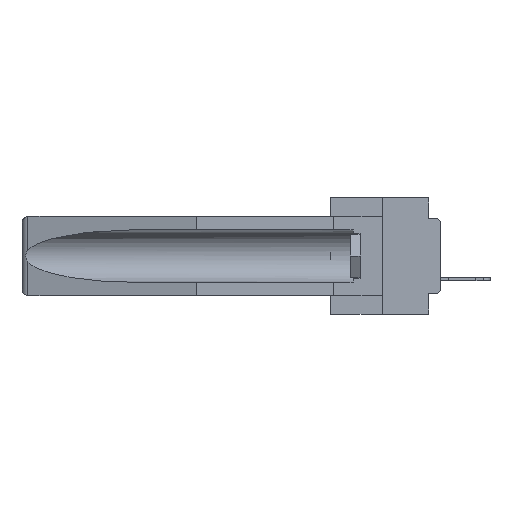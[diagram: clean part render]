
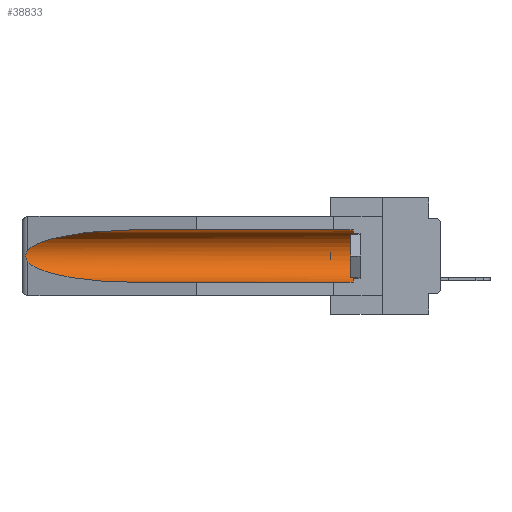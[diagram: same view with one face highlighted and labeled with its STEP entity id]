
A CAD part, left-side view. The second image highlights one B-rep face of the part: STEP entity #38833.
In plain terms, the highlighted cylindrical face has radius 2.857 mm (diameter 5.715 mm), a partial arc.
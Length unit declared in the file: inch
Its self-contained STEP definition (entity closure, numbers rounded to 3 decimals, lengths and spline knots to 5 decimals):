
#16 = LINE ( 'NONE', #34890, #8395 ) ;
#992 = CARTESIAN_POINT ( 'NONE',  ( 0.155, 0.126, -0.1715 ) ) ;
#1209 = EDGE_CURVE ( 'NONE', #10448, #9523, #7108, .T. ) ;
#2883 = VERTEX_POINT ( 'NONE', #7000 ) ;
#3504 = CARTESIAN_POINT ( 'NONE',  ( 0.25451, 1.48313, -0.09465 ) ) ;
#4136 = ORIENTED_EDGE ( 'NONE', *, *, #5567, .T. ) ;
#4322 = CARTESIAN_POINT ( 'NONE',  ( 0.26654, 1.53092, -0.15636 ) ) ;
#4549 = VECTOR ( 'NONE', #17404, 39.37008 ) ;
#5567 = EDGE_CURVE ( 'NONE', #2883, #10448, #33240, .T. ) ;
#6249 = DIRECTION ( 'NONE',  ( 0., 0., 1. ) ) ;
#6333 = VERTEX_POINT ( 'NONE', #38451 ) ;
#6442 = ORIENTED_EDGE ( 'NONE', *, *, #27187, .T. ) ;
#6509 = CARTESIAN_POINT ( 'NONE',  ( 0.155, -0.30754, -0.1715 ) ) ;
#7000 = CARTESIAN_POINT ( 'NONE',  ( 0.155, 1.07973, -0.059 ) ) ;
#7108 = B_SPLINE_CURVE_WITH_KNOTS ( 'NONE', 3,
 ( #26127, #9974, #4322, #22998, #35329, #26265, #19696, #31904, #32037, #7487 ),
 .UNSPECIFIED., .F., .F.,
 ( 4, 2, 2, 2, 4 ),
 ( 0., 0.00029, 0.00058, 0.00087, 0.00117 ),
 .UNSPECIFIED. ) ;
#7487 = CARTESIAN_POINT ( 'NONE',  ( 0.26537, 1.52718, -0.19328 ) ) ;
#7825 = CARTESIAN_POINT ( 'NONE',  ( 0.155, -0.30754, -0.059 ) ) ;
#8395 = VECTOR ( 'NONE', #31593, 39.37008 ) ;
#9523 = VERTEX_POINT ( 'NONE', #29130 ) ;
#9845 = CARTESIAN_POINT ( 'NONE',  ( 0.26537, 1.52718, -0.14972 ) ) ;
#9974 = CARTESIAN_POINT ( 'NONE',  ( 0.26597, 1.52961, -0.15275 ) ) ;
#10448 = VERTEX_POINT ( 'NONE', #27277 ) ;
#11919 = LINE ( 'NONE', #7825, #4549 ) ;
#12287 = EDGE_LOOP ( 'NONE', ( #4136, #14485, #6442, #29864, #29641, #24437 ) ) ;
#12651 =( BOUNDED_CURVE ( )  B_SPLINE_CURVE ( 3, ( #26542, #36136, #26671, #23794 ),
 .UNSPECIFIED., .F., .T. ) 
 B_SPLINE_CURVE_WITH_KNOTS ( ( 4, 4 ),
 ( 0.1948, 1.5708 ),
 .UNSPECIFIED. ) 
 CURVE ( )  GEOMETRIC_REPRESENTATION_ITEM ( )  RATIONAL_B_SPLINE_CURVE ( ( 1., 0.848, 0.848, 1. ) ) 
 REPRESENTATION_ITEM ( '' )  );
#13105 = DIRECTION ( 'NONE',  ( 0., -1., 0. ) ) ;
#14485 = ORIENTED_EDGE ( 'NONE', *, *, #1209, .T. ) ;
#14990 = AXIS2_PLACEMENT_3D ( 'NONE', #6509, #37930, #6249 ) ;
#15881 = CARTESIAN_POINT ( 'NONE',  ( 0.21114, 1.30732, -0.059 ) ) ;
#16428 = CARTESIAN_POINT ( 'NONE',  ( 0.155, 0.126, -0.059 ) ) ;
#17404 = DIRECTION ( 'NONE',  ( 0., 1., 0. ) ) ;
#17906 = AXIS2_PLACEMENT_3D ( 'NONE', #992, #13105, #38048 ) ;
#18976 = VERTEX_POINT ( 'NONE', #31317 ) ;
#19696 = CARTESIAN_POINT ( 'NONE',  ( 0.2673, 1.53269, -0.17917 ) ) ;
#22998 = CARTESIAN_POINT ( 'NONE',  ( 0.2673, 1.5327, -0.16383 ) ) ;
#23794 = CARTESIAN_POINT ( 'NONE',  ( 0.155, 1.07973, -0.284 ) ) ;
#24437 = ORIENTED_EDGE ( 'NONE', *, *, #39695, .T. ) ;
#25573 = EDGE_CURVE ( 'NONE', #6333, #18976, #16, .T. ) ;
#26127 = CARTESIAN_POINT ( 'NONE',  ( 0.26537, 1.52718, -0.14972 ) ) ;
#26265 = CARTESIAN_POINT ( 'NONE',  ( 0.2675, 1.53308, -0.17534 ) ) ;
#26542 = CARTESIAN_POINT ( 'NONE',  ( 0.26537, 1.52718, -0.19328 ) ) ;
#26671 = CARTESIAN_POINT ( 'NONE',  ( 0.21114, 1.30732, -0.284 ) ) ;
#27187 = EDGE_CURVE ( 'NONE', #9523, #18976, #12651, .T. ) ;
#27277 = CARTESIAN_POINT ( 'NONE',  ( 0.26537, 1.52718, -0.14972 ) ) ;
#29130 = CARTESIAN_POINT ( 'NONE',  ( 0.26537, 1.52718, -0.19328 ) ) ;
#29607 = CYLINDRICAL_SURFACE ( 'NONE', #14990, 0.1125 ) ;
#29641 = ORIENTED_EDGE ( 'NONE', *, *, #40691, .T. ) ;
#29864 = ORIENTED_EDGE ( 'NONE', *, *, #25573, .F. ) ;
#30593 = FACE_OUTER_BOUND ( 'NONE', #12287, .T. ) ;
#31317 = CARTESIAN_POINT ( 'NONE',  ( 0.155, 1.07973, -0.284 ) ) ;
#31593 = DIRECTION ( 'NONE',  ( 0., 1., 0. ) ) ;
#31904 = CARTESIAN_POINT ( 'NONE',  ( 0.26655, 1.53094, -0.18657 ) ) ;
#32037 = CARTESIAN_POINT ( 'NONE',  ( 0.26597, 1.5296, -0.19026 ) ) ;
#33061 = VERTEX_POINT ( 'NONE', #16428 ) ;
#33240 =( BOUNDED_CURVE ( )  B_SPLINE_CURVE ( 3, ( #35071, #15881, #3504, #9845 ),
 .UNSPECIFIED., .F., .T. ) 
 B_SPLINE_CURVE_WITH_KNOTS ( ( 4, 4 ),
 ( 4.71239, 6.08839 ),
 .UNSPECIFIED. ) 
 CURVE ( )  GEOMETRIC_REPRESENTATION_ITEM ( )  RATIONAL_B_SPLINE_CURVE ( ( 1., 0.848, 0.848, 1. ) ) 
 REPRESENTATION_ITEM ( '' )  );
#34484 = CIRCLE ( 'NONE', #17906, 0.1125 ) ;
#34890 = CARTESIAN_POINT ( 'NONE',  ( 0.155, -0.30754, -0.284 ) ) ;
#35071 = CARTESIAN_POINT ( 'NONE',  ( 0.155, 1.07973, -0.059 ) ) ;
#35329 = CARTESIAN_POINT ( 'NONE',  ( 0.2675, 1.53308, -0.16763 ) ) ;
#36136 = CARTESIAN_POINT ( 'NONE',  ( 0.25451, 1.48313, -0.24835 ) ) ;
#37930 = DIRECTION ( 'NONE',  ( 0., 1., 0. ) ) ;
#38048 = DIRECTION ( 'NONE',  ( 0., 0., 1. ) ) ;
#38451 = CARTESIAN_POINT ( 'NONE',  ( 0.155, 0.126, -0.284 ) ) ;
#38833 = ADVANCED_FACE ( 'NONE', ( #30593 ), #29607, .F. ) ;
#39695 = EDGE_CURVE ( 'NONE', #33061, #2883, #11919, .T. ) ;
#40691 = EDGE_CURVE ( 'NONE', #6333, #33061, #34484, .T. ) ;
